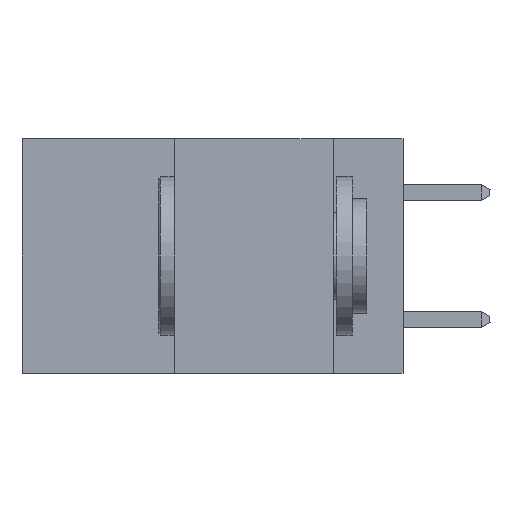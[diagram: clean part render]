
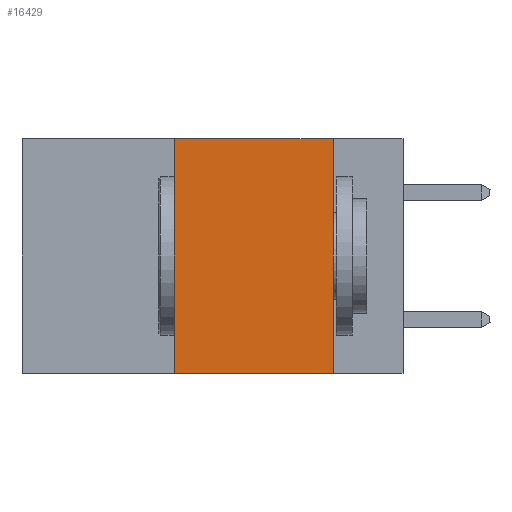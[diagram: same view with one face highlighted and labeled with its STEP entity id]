
A CAD part, left-side view. The second image highlights one B-rep face of the part: STEP entity #16429.
In plain terms, the highlighted planar face has unit normal (-1, 0, 0).
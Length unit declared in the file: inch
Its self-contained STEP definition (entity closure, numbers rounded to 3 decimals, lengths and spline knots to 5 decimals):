
#807 = EDGE_CURVE ( 'NONE', #22453, #38496, #15473, .T. ) ;
#3642 = LINE ( 'NONE', #15896, #24274 ) ;
#5494 = CARTESIAN_POINT ( 'NONE',  ( 0., 0.36, -0.37 ) ) ;
#9693 = PLANE ( 'NONE',  #14255 ) ;
#10484 = CARTESIAN_POINT ( 'NONE',  ( 0., 0.11, 0. ) ) ;
#10665 = EDGE_CURVE ( 'NONE', #38496, #14653, #13994, .T. ) ;
#10714 = EDGE_CURVE ( 'NONE', #14653, #16522, #3642, .T. ) ;
#12008 = FACE_OUTER_BOUND ( 'NONE', #24743, .T. ) ;
#13994 = LINE ( 'NONE', #28676, #24823 ) ;
#14255 = AXIS2_PLACEMENT_3D ( 'NONE', #20145, #37366, #37232 ) ;
#14653 = VERTEX_POINT ( 'NONE', #10484 ) ;
#14700 = ORIENTED_EDGE ( 'NONE', *, *, #26193, .T. ) ;
#15473 = LINE ( 'NONE', #27906, #19322 ) ;
#15896 = CARTESIAN_POINT ( 'NONE',  ( 0., 0.11, 0. ) ) ;
#16429 = ADVANCED_FACE ( 'NONE', ( #12008 ), #9693, .F. ) ;
#16522 = VERTEX_POINT ( 'NONE', #41755 ) ;
#18846 = DIRECTION ( 'NONE',  ( 0., -1., 0. ) ) ;
#19322 = VECTOR ( 'NONE', #34952, 39.37008 ) ;
#19904 = CARTESIAN_POINT ( 'NONE',  ( 0., 0.36, 0. ) ) ;
#20145 = CARTESIAN_POINT ( 'NONE',  ( 0., 0.6, 0. ) ) ;
#21878 = CARTESIAN_POINT ( 'NONE',  ( 0., 0.6, -0.37 ) ) ;
#22453 = VERTEX_POINT ( 'NONE', #5494 ) ;
#22598 = DIRECTION ( 'NONE',  ( 0., 0., -1. ) ) ;
#23042 = LINE ( 'NONE', #21878, #26295 ) ;
#24274 = VECTOR ( 'NONE', #22598, 39.37008 ) ;
#24743 = EDGE_LOOP ( 'NONE', ( #35252, #42584, #41156, #14700 ) ) ;
#24823 = VECTOR ( 'NONE', #32746, 39.37008 ) ;
#26193 = EDGE_CURVE ( 'NONE', #22453, #16522, #23042, .T. ) ;
#26295 = VECTOR ( 'NONE', #18846, 39.37008 ) ;
#27906 = CARTESIAN_POINT ( 'NONE',  ( 0., 0.36, 0. ) ) ;
#28676 = CARTESIAN_POINT ( 'NONE',  ( 0., 0.6, 0. ) ) ;
#32746 = DIRECTION ( 'NONE',  ( 0., -1., 0. ) ) ;
#34952 = DIRECTION ( 'NONE',  ( 0., 0., 1. ) ) ;
#35252 = ORIENTED_EDGE ( 'NONE', *, *, #10714, .F. ) ;
#37232 = DIRECTION ( 'NONE',  ( 0., 0., -1. ) ) ;
#37366 = DIRECTION ( 'NONE',  ( 1., 0., 0. ) ) ;
#38496 = VERTEX_POINT ( 'NONE', #19904 ) ;
#41156 = ORIENTED_EDGE ( 'NONE', *, *, #807, .F. ) ;
#41755 = CARTESIAN_POINT ( 'NONE',  ( 0., 0.11, -0.37 ) ) ;
#42584 = ORIENTED_EDGE ( 'NONE', *, *, #10665, .F. ) ;
